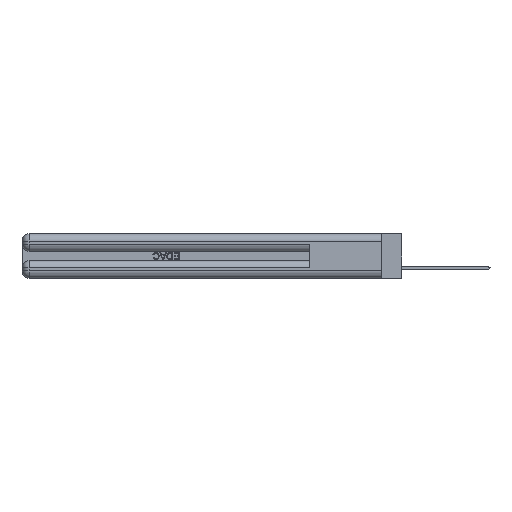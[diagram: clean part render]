
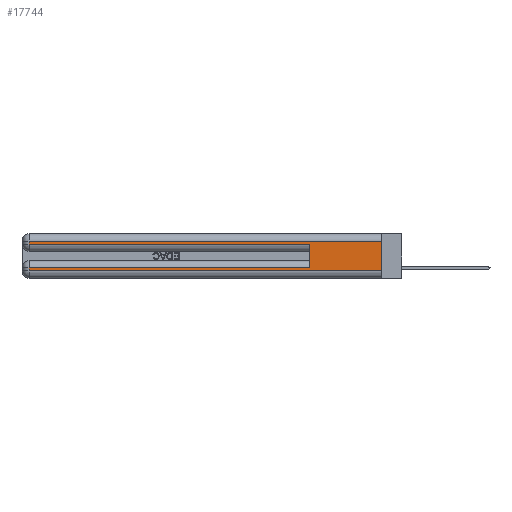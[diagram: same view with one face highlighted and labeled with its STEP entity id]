
A CAD part, left-side view. The second image highlights one B-rep face of the part: STEP entity #17744.
In plain terms, the highlighted planar face has unit normal (-1, 0, 0).
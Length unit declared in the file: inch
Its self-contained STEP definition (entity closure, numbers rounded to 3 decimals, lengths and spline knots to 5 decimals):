
#31 = VERTEX_POINT ( 'NONE', #35104 ) ;
#1353 = DIRECTION ( 'NONE',  ( 0., 0., 1. ) ) ;
#1607 = DIRECTION ( 'NONE',  ( 0., -1., 0. ) ) ;
#2267 = ORIENTED_EDGE ( 'NONE', *, *, #27334, .T. ) ;
#2285 = AXIS2_PLACEMENT_3D ( 'NONE', #37402, #14393, #37560 ) ;
#2765 = DIRECTION ( 'NONE',  ( 0., 0., -1. ) ) ;
#3069 = VECTOR ( 'NONE', #46167, 39.37008 ) ;
#4821 = DIRECTION ( 'NONE',  ( 0., 1., 0. ) ) ;
#5327 = LINE ( 'NONE', #13140, #46831 ) ;
#6192 = CARTESIAN_POINT ( 'NONE',  ( 0., 2.94, 0.37 ) ) ;
#6225 = CARTESIAN_POINT ( 'NONE',  ( 0., 0., 0.31 ) ) ;
#6242 = EDGE_CURVE ( 'NONE', #29846, #48520, #40998, .T. ) ;
#7142 = LINE ( 'NONE', #46331, #39692 ) ;
#9430 = ORIENTED_EDGE ( 'NONE', *, *, #6242, .T. ) ;
#9754 = ORIENTED_EDGE ( 'NONE', *, *, #36353, .T. ) ;
#10302 = VERTEX_POINT ( 'NONE', #45561 ) ;
#10318 = CARTESIAN_POINT ( 'NONE',  ( 0., 0.6, 0.085 ) ) ;
#10497 = VECTOR ( 'NONE', #2765, 39.37008 ) ;
#10875 = ORIENTED_EDGE ( 'NONE', *, *, #36858, .T. ) ;
#11884 = CARTESIAN_POINT ( 'NONE',  ( 0., 2.94, 0.37 ) ) ;
#12138 = LINE ( 'NONE', #11884, #21685 ) ;
#12254 = CARTESIAN_POINT ( 'NONE',  ( 0., 0., 0.085 ) ) ;
#12413 = ORIENTED_EDGE ( 'NONE', *, *, #27956, .T. ) ;
#13140 = CARTESIAN_POINT ( 'NONE',  ( 0., 0.6, 0.145 ) ) ;
#13340 = ORIENTED_EDGE ( 'NONE', *, *, #40400, .T. ) ;
#13756 = CARTESIAN_POINT ( 'NONE',  ( 0., 0., 0.285 ) ) ;
#14393 = DIRECTION ( 'NONE',  ( 1., 0., 0. ) ) ;
#15086 = VERTEX_POINT ( 'NONE', #45239 ) ;
#15090 = VERTEX_POINT ( 'NONE', #19763 ) ;
#15859 = LINE ( 'NONE', #12254, #28975 ) ;
#17744 = ADVANCED_FACE ( 'NONE', ( #20686 ), #29783, .F. ) ;
#19763 = CARTESIAN_POINT ( 'NONE',  ( 0., 2.94, 0.085 ) ) ;
#20686 = FACE_OUTER_BOUND ( 'NONE', #43099, .T. ) ;
#21685 = VECTOR ( 'NONE', #35071, 39.37008 ) ;
#22742 = VECTOR ( 'NONE', #44260, 39.37008 ) ;
#24593 = LINE ( 'NONE', #6225, #44807 ) ;
#24785 = CARTESIAN_POINT ( 'NONE',  ( 0., 0., 0.37 ) ) ;
#27334 = EDGE_CURVE ( 'NONE', #10302, #29846, #24593, .T. ) ;
#27956 = EDGE_CURVE ( 'NONE', #48520, #45980, #32807, .T. ) ;
#28427 = ORIENTED_EDGE ( 'NONE', *, *, #35181, .F. ) ;
#28789 = CARTESIAN_POINT ( 'NONE',  ( 0., 2.94, 0.31 ) ) ;
#28975 = VECTOR ( 'NONE', #4821, 39.37008 ) ;
#29783 = PLANE ( 'NONE',  #2285 ) ;
#29846 = VERTEX_POINT ( 'NONE', #28789 ) ;
#31766 = LINE ( 'NONE', #24785, #10497 ) ;
#32689 = DIRECTION ( 'NONE',  ( 0., 1., 0. ) ) ;
#32807 = LINE ( 'NONE', #13756, #22742 ) ;
#33167 = CARTESIAN_POINT ( 'NONE',  ( 0., 2.94, 0.285 ) ) ;
#35071 = DIRECTION ( 'NONE',  ( 0., 0., -1. ) ) ;
#35104 = CARTESIAN_POINT ( 'NONE',  ( 0., 2.94, 0.06 ) ) ;
#35181 = EDGE_CURVE ( 'NONE', #35202, #45980, #5327, .T. ) ;
#35202 = VERTEX_POINT ( 'NONE', #10318 ) ;
#36353 = EDGE_CURVE ( 'NONE', #35202, #15090, #15859, .T. ) ;
#36858 = EDGE_CURVE ( 'NONE', #15090, #31, #12138, .T. ) ;
#37402 = CARTESIAN_POINT ( 'NONE',  ( 0., 0., 0.37 ) ) ;
#37560 = DIRECTION ( 'NONE',  ( 0., 0., -1. ) ) ;
#39692 = VECTOR ( 'NONE', #1607, 39.37008 ) ;
#40400 = EDGE_CURVE ( 'NONE', #31, #15086, #7142, .T. ) ;
#40998 = LINE ( 'NONE', #6192, #3069 ) ;
#42096 = EDGE_CURVE ( 'NONE', #10302, #15086, #31766, .T. ) ;
#43099 = EDGE_LOOP ( 'NONE', ( #45327, #2267, #9430, #12413, #28427, #9754, #10875, #13340 ) ) ;
#44260 = DIRECTION ( 'NONE',  ( 0., -1., 0. ) ) ;
#44807 = VECTOR ( 'NONE', #32689, 39.37008 ) ;
#45239 = CARTESIAN_POINT ( 'NONE',  ( 0., 0., 0.06 ) ) ;
#45327 = ORIENTED_EDGE ( 'NONE', *, *, #42096, .F. ) ;
#45561 = CARTESIAN_POINT ( 'NONE',  ( 0., 0., 0.31 ) ) ;
#45980 = VERTEX_POINT ( 'NONE', #46039 ) ;
#46039 = CARTESIAN_POINT ( 'NONE',  ( 0., 0.6, 0.285 ) ) ;
#46167 = DIRECTION ( 'NONE',  ( 0., 0., -1. ) ) ;
#46331 = CARTESIAN_POINT ( 'NONE',  ( 0., 0., 0.06 ) ) ;
#46831 = VECTOR ( 'NONE', #1353, 39.37008 ) ;
#48520 = VERTEX_POINT ( 'NONE', #33167 ) ;
